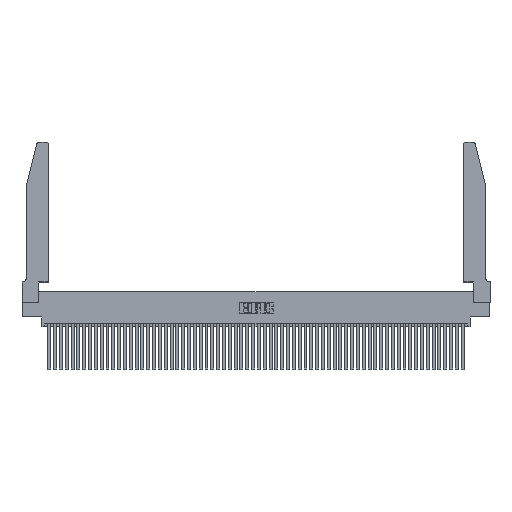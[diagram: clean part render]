
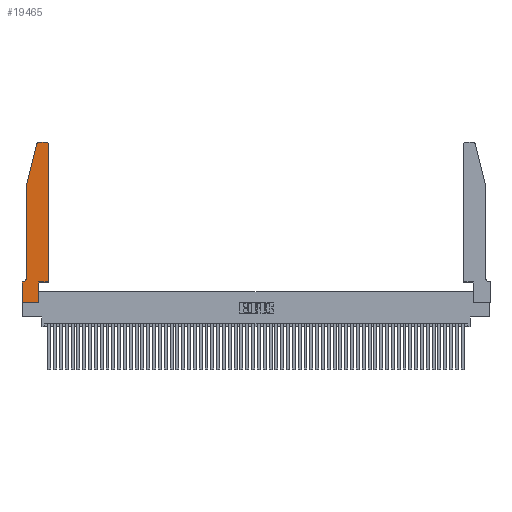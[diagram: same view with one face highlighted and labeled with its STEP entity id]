
A CAD part, top view. The second image highlights one B-rep face of the part: STEP entity #19465.
In plain terms, the highlighted planar face has unit normal (0, 0, 1).
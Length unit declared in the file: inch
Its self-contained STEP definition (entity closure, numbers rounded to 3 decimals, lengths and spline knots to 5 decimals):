
#273 = CARTESIAN_POINT ( 'NONE',  ( 0.4505, 0.35, 0.37 ) ) ;
#373 = DIRECTION ( 'NONE',  ( 0., 0., 1. ) ) ;
#437 = VECTOR ( 'NONE', #51713, 39.37008 ) ;
#1318 = EDGE_CURVE ( 'NONE', #10040, #50826, #44191, .T. ) ;
#1394 = EDGE_CURVE ( 'NONE', #34599, #16571, #18128, .T. ) ;
#3367 = AXIS2_PLACEMENT_3D ( 'NONE', #16007, #46664, #20465 ) ;
#3596 = CARTESIAN_POINT ( 'NONE',  ( 0., 0., 0.37 ) ) ;
#3933 = DIRECTION ( 'NONE',  ( -1., 0., 0. ) ) ;
#4109 = EDGE_CURVE ( 'NONE', #34306, #35540, #14345, .T. ) ;
#4720 = VECTOR ( 'NONE', #3933, 39.37008 ) ;
#5197 = VERTEX_POINT ( 'NONE', #18841 ) ;
#5228 = ORIENTED_EDGE ( 'NONE', *, *, #15984, .T. ) ;
#5464 = ORIENTED_EDGE ( 'NONE', *, *, #41837, .T. ) ;
#5859 = CARTESIAN_POINT ( 'NONE',  ( 0.0755, 2., 0.37 ) ) ;
#6181 = VECTOR ( 'NONE', #54393, 39.37008 ) ;
#7198 = DIRECTION ( 'NONE',  ( 0., 1., 0. ) ) ;
#8175 = DIRECTION ( 'NONE',  ( 0., -1., 0. ) ) ;
#8345 = CARTESIAN_POINT ( 'NONE',  ( 0.2865, 0.35, 0.37 ) ) ;
#9138 = CARTESIAN_POINT ( 'NONE',  ( 0.4205, 2.72, 0.37 ) ) ;
#10040 = VERTEX_POINT ( 'NONE', #26767 ) ;
#12177 = CARTESIAN_POINT ( 'NONE',  ( 0., 0., 0.37 ) ) ;
#12463 = EDGE_CURVE ( 'NONE', #5197, #10040, #12503, .T. ) ;
#12503 = LINE ( 'NONE', #12177, #437 ) ;
#12914 = ORIENTED_EDGE ( 'NONE', *, *, #47660, .T. ) ;
#13312 = ORIENTED_EDGE ( 'NONE', *, *, #12463, .T. ) ;
#13439 = CARTESIAN_POINT ( 'NONE',  ( 0.25487, 2.72718, 0.37 ) ) ;
#13672 = DIRECTION ( 'NONE',  ( 1., 0., 0. ) ) ;
#14115 = DIRECTION ( 'NONE',  ( 1., 0., 0. ) ) ;
#14345 = LINE ( 'NONE', #33955, #36355 ) ;
#15984 = EDGE_CURVE ( 'NONE', #35540, #45011, #32892, .T. ) ;
#16007 = CARTESIAN_POINT ( 'NONE',  ( 0., 0.35, 0.37 ) ) ;
#16243 = EDGE_CURVE ( 'NONE', #25613, #5197, #53995, .T. ) ;
#16470 = DIRECTION ( 'NONE',  ( 0., 0., -1. ) ) ;
#16571 = VERTEX_POINT ( 'NONE', #32569 ) ;
#16674 = DIRECTION ( 'NONE',  ( -0.239, -0.971, 0. ) ) ;
#17327 = ORIENTED_EDGE ( 'NONE', *, *, #16243, .T. ) ;
#17611 = AXIS2_PLACEMENT_3D ( 'NONE', #9138, #39978, #13672 ) ;
#18128 = LINE ( 'NONE', #5859, #6181 ) ;
#18841 = CARTESIAN_POINT ( 'NONE',  ( 0., 0., 0.37 ) ) ;
#18929 = ORIENTED_EDGE ( 'NONE', *, *, #31897, .T. ) ;
#19019 = CARTESIAN_POINT ( 'NONE',  ( 0.2865, 0.35, 0.37 ) ) ;
#19465 = ADVANCED_FACE ( 'NONE', ( #52733 ), #20271, .T. ) ;
#19707 = CARTESIAN_POINT ( 'NONE',  ( 0., 0.35, 0.37 ) ) ;
#19971 = VERTEX_POINT ( 'NONE', #49463 ) ;
#20042 = ORIENTED_EDGE ( 'NONE', *, *, #4109, .T. ) ;
#20271 = PLANE ( 'NONE',  #3367 ) ;
#20465 = DIRECTION ( 'NONE',  ( 1., 0., 0. ) ) ;
#20690 = CARTESIAN_POINT ( 'NONE',  ( 0.4205, 2.75, 0.37 ) ) ;
#20942 = VECTOR ( 'NONE', #40854, 39.37008 ) ;
#23411 = EDGE_LOOP ( 'NONE', ( #5464, #38025, #39046, #45165, #23843, #12914, #17327, #13312, #33464, #18929, #20042, #5228 ) ) ;
#23843 = ORIENTED_EDGE ( 'NONE', *, *, #41162, .T. ) ;
#24215 = CARTESIAN_POINT ( 'NONE',  ( 0.4505, 2.72, 0.37 ) ) ;
#25613 = VERTEX_POINT ( 'NONE', #19707 ) ;
#26101 = CARTESIAN_POINT ( 'NONE',  ( 0.2605, 2.75, 0.37 ) ) ;
#26767 = CARTESIAN_POINT ( 'NONE',  ( 0.2865, 0., 0.37 ) ) ;
#27190 = CARTESIAN_POINT ( 'NONE',  ( 0.284, 2.72, 0.37 ) ) ;
#27906 = EDGE_CURVE ( 'NONE', #53155, #43473, #51360, .T. ) ;
#28058 = LINE ( 'NONE', #47310, #29416 ) ;
#28660 = AXIS2_PLACEMENT_3D ( 'NONE', #27190, #373, #31576 ) ;
#29416 = VECTOR ( 'NONE', #16674, 39.37008 ) ;
#30633 = VECTOR ( 'NONE', #14115, 39.37008 ) ;
#31576 = DIRECTION ( 'NONE',  ( 1., 0., 0. ) ) ;
#31897 = EDGE_CURVE ( 'NONE', #50826, #34306, #55217, .T. ) ;
#32417 = CARTESIAN_POINT ( 'NONE',  ( 0.4505, 0.35, 0.37 ) ) ;
#32569 = CARTESIAN_POINT ( 'NONE',  ( 0.0755, 0.42, 0.37 ) ) ;
#32892 = CIRCLE ( 'NONE', #17611, 0.03 ) ;
#33464 = ORIENTED_EDGE ( 'NONE', *, *, #1318, .T. ) ;
#33955 = CARTESIAN_POINT ( 'NONE',  ( 0.4505, 0.35, 0.37 ) ) ;
#34306 = VERTEX_POINT ( 'NONE', #32417 ) ;
#34599 = VERTEX_POINT ( 'NONE', #47997 ) ;
#35014 = CARTESIAN_POINT ( 'NONE',  ( 0.0755, 0.35, 0.37 ) ) ;
#35540 = VERTEX_POINT ( 'NONE', #24215 ) ;
#35624 = VECTOR ( 'NONE', #39237, 39.37008 ) ;
#36355 = VECTOR ( 'NONE', #7198, 39.37008 ) ;
#38025 = ORIENTED_EDGE ( 'NONE', *, *, #27906, .T. ) ;
#38187 = AXIS2_PLACEMENT_3D ( 'NONE', #42751, #16470, #47113 ) ;
#39046 = ORIENTED_EDGE ( 'NONE', *, *, #44430, .T. ) ;
#39237 = DIRECTION ( 'NONE',  ( -1., 0., 0. ) ) ;
#39978 = DIRECTION ( 'NONE',  ( 0., 0., 1. ) ) ;
#40763 = CARTESIAN_POINT ( 'NONE',  ( 0.284, 2.75, 0.37 ) ) ;
#40854 = DIRECTION ( 'NONE',  ( 0., 1., 0. ) ) ;
#41162 = EDGE_CURVE ( 'NONE', #16571, #19971, #56864, .T. ) ;
#41837 = EDGE_CURVE ( 'NONE', #45011, #53155, #47215, .T. ) ;
#42403 = VECTOR ( 'NONE', #8175, 39.37008 ) ;
#42751 = CARTESIAN_POINT ( 'NONE',  ( 0.0055, 0.42, 0.37 ) ) ;
#43473 = VERTEX_POINT ( 'NONE', #13439 ) ;
#44191 = LINE ( 'NONE', #19019, #20942 ) ;
#44430 = EDGE_CURVE ( 'NONE', #43473, #34599, #28058, .T. ) ;
#45011 = VERTEX_POINT ( 'NONE', #20690 ) ;
#45165 = ORIENTED_EDGE ( 'NONE', *, *, #1394, .T. ) ;
#46664 = DIRECTION ( 'NONE',  ( 0., 0., 1. ) ) ;
#47113 = DIRECTION ( 'NONE',  ( -1., 0., 0. ) ) ;
#47215 = LINE ( 'NONE', #26101, #35624 ) ;
#47310 = CARTESIAN_POINT ( 'NONE',  ( 0.0755, 2., 0.37 ) ) ;
#47660 = EDGE_CURVE ( 'NONE', #19971, #25613, #48907, .T. ) ;
#47997 = CARTESIAN_POINT ( 'NONE',  ( 0.0755, 2., 0.37 ) ) ;
#48907 = LINE ( 'NONE', #35014, #4720 ) ;
#49463 = CARTESIAN_POINT ( 'NONE',  ( 0.0055, 0.35, 0.37 ) ) ;
#50826 = VERTEX_POINT ( 'NONE', #8345 ) ;
#51360 = CIRCLE ( 'NONE', #28660, 0.03 ) ;
#51713 = DIRECTION ( 'NONE',  ( 1., 0., 0. ) ) ;
#52733 = FACE_OUTER_BOUND ( 'NONE', #23411, .T. ) ;
#53155 = VERTEX_POINT ( 'NONE', #40763 ) ;
#53995 = LINE ( 'NONE', #3596, #42403 ) ;
#54393 = DIRECTION ( 'NONE',  ( 0., -1., 0. ) ) ;
#55217 = LINE ( 'NONE', #273, #30633 ) ;
#56864 = CIRCLE ( 'NONE', #38187, 0.07 ) ;
